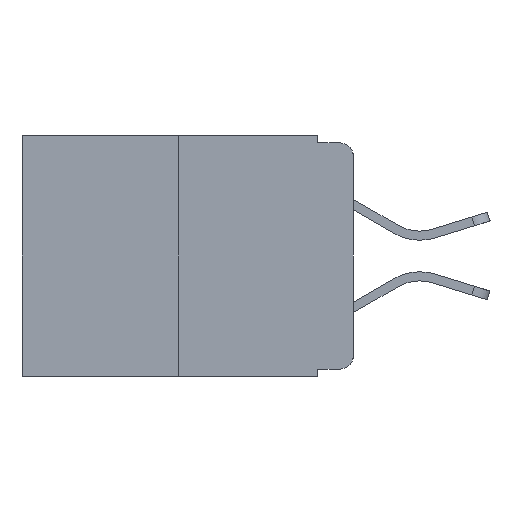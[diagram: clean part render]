
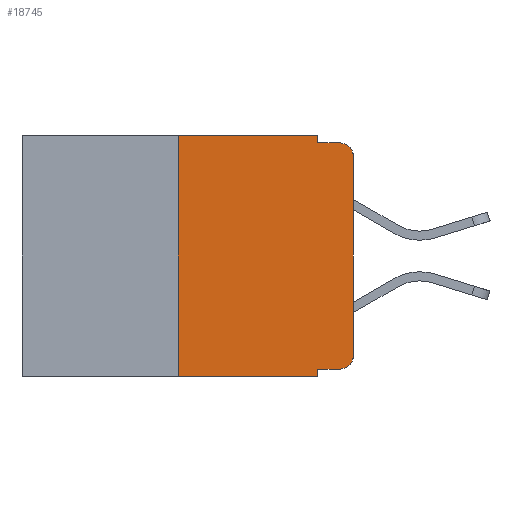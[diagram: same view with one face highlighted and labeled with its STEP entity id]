
A CAD part, left-side view. The second image highlights one B-rep face of the part: STEP entity #18745.
In plain terms, the highlighted planar face has unit normal (-1, 0, 0).
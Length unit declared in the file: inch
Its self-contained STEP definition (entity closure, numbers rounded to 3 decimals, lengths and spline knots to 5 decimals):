
#181 = EDGE_CURVE ( 'NONE', #6180, #10598, #3139, .T. ) ;
#533 = EDGE_CURVE ( 'NONE', #6180, #20550, #6608, .T. ) ;
#753 = LINE ( 'NONE', #8693, #20021 ) ;
#947 = DIRECTION ( 'NONE',  ( 0., 0., -1. ) ) ;
#1002 = ORIENTED_EDGE ( 'NONE', *, *, #10294, .T. ) ;
#1076 = VERTEX_POINT ( 'NONE', #17053 ) ;
#1227 = CARTESIAN_POINT ( 'NONE',  ( 0., 0.02, -0.313 ) ) ;
#2533 = CARTESIAN_POINT ( 'NONE',  ( 0., 0.051, 0. ) ) ;
#2749 = EDGE_CURVE ( 'NONE', #11808, #15245, #6987, .T. ) ;
#2962 = DIRECTION ( 'NONE',  ( 0., 0., 1. ) ) ;
#3079 = ORIENTED_EDGE ( 'NONE', *, *, #6478, .F. ) ;
#3130 = DIRECTION ( 'NONE',  ( 0., 0., -1. ) ) ;
#3139 = LINE ( 'NONE', #13725, #12553 ) ;
#3158 = AXIS2_PLACEMENT_3D ( 'NONE', #1227, #14376, #3130 ) ;
#3299 = LINE ( 'NONE', #3784, #22401 ) ;
#3784 = CARTESIAN_POINT ( 'NONE',  ( 0., 0.051, -0.01 ) ) ;
#4069 = LINE ( 'NONE', #22769, #8427 ) ;
#4880 = VECTOR ( 'NONE', #19027, 39.37008 ) ;
#5183 = DIRECTION ( 'NONE',  ( 0., 0., 1. ) ) ;
#6013 = ORIENTED_EDGE ( 'NONE', *, *, #20651, .T. ) ;
#6180 = VERTEX_POINT ( 'NONE', #21287 ) ;
#6381 = CARTESIAN_POINT ( 'NONE',  ( 0., 0.473, -0.343 ) ) ;
#6478 = EDGE_CURVE ( 'NONE', #15245, #23423, #3299, .T. ) ;
#6608 = LINE ( 'NONE', #6381, #4880 ) ;
#6987 = LINE ( 'NONE', #8072, #21183 ) ;
#7202 = ORIENTED_EDGE ( 'NONE', *, *, #23045, .F. ) ;
#8015 = DIRECTION ( 'NONE',  ( 0., 0., -1. ) ) ;
#8072 = CARTESIAN_POINT ( 'NONE',  ( 0., 0.051, 0. ) ) ;
#8427 = VECTOR ( 'NONE', #11898, 39.37008 ) ;
#8604 = CARTESIAN_POINT ( 'NONE',  ( 0., 0.051, -0.343 ) ) ;
#8693 = CARTESIAN_POINT ( 'NONE',  ( 0., 0.473, 0. ) ) ;
#8812 = AXIS2_PLACEMENT_3D ( 'NONE', #23156, #12225, #947 ) ;
#8959 = ORIENTED_EDGE ( 'NONE', *, *, #14393, .F. ) ;
#9006 = EDGE_CURVE ( 'NONE', #16203, #23423, #22796, .T. ) ;
#9014 = CIRCLE ( 'NONE', #3158, 0.02 ) ;
#9024 = CARTESIAN_POINT ( 'NONE',  ( 0., 0., -0.313 ) ) ;
#9317 = CARTESIAN_POINT ( 'NONE',  ( 0., 0.051, -0.01 ) ) ;
#9419 = FACE_OUTER_BOUND ( 'NONE', #19785, .T. ) ;
#9778 = VECTOR ( 'NONE', #2962, 39.37008 ) ;
#10030 = VERTEX_POINT ( 'NONE', #18888 ) ;
#10080 = PLANE ( 'NONE',  #20150 ) ;
#10155 = CARTESIAN_POINT ( 'NONE',  ( 0., 0.473, 0. ) ) ;
#10159 = ORIENTED_EDGE ( 'NONE', *, *, #2749, .F. ) ;
#10294 = EDGE_CURVE ( 'NONE', #16328, #16203, #20779, .T. ) ;
#10598 = VERTEX_POINT ( 'NONE', #23136 ) ;
#11808 = VERTEX_POINT ( 'NONE', #2533 ) ;
#11898 = DIRECTION ( 'NONE',  ( 0., -1., 0. ) ) ;
#12061 = DIRECTION ( 'NONE',  ( 0., 0., -1. ) ) ;
#12225 = DIRECTION ( 'NONE',  ( -1., 0., 0. ) ) ;
#12337 = CARTESIAN_POINT ( 'NONE',  ( 0., 0., 0. ) ) ;
#12519 = DIRECTION ( 'NONE',  ( 0., -1., 0. ) ) ;
#12553 = VECTOR ( 'NONE', #5183, 39.37008 ) ;
#12586 = CARTESIAN_POINT ( 'NONE',  ( 0., 0.02, -0.01 ) ) ;
#12827 = ORIENTED_EDGE ( 'NONE', *, *, #533, .T. ) ;
#13489 = DIRECTION ( 'NONE',  ( 0., 0., -1. ) ) ;
#13725 = CARTESIAN_POINT ( 'NONE',  ( 0., 0.25, 0. ) ) ;
#14376 = DIRECTION ( 'NONE',  ( -1., 0., 0. ) ) ;
#14393 = EDGE_CURVE ( 'NONE', #10598, #11808, #753, .T. ) ;
#15245 = VERTEX_POINT ( 'NONE', #9317 ) ;
#16203 = VERTEX_POINT ( 'NONE', #21548 ) ;
#16328 = VERTEX_POINT ( 'NONE', #9024 ) ;
#17053 = CARTESIAN_POINT ( 'NONE',  ( 0., 0.02, -0.333 ) ) ;
#17437 = VECTOR ( 'NONE', #13489, 39.37008 ) ;
#17756 = ORIENTED_EDGE ( 'NONE', *, *, #181, .F. ) ;
#18009 = LINE ( 'NONE', #20763, #17437 ) ;
#18250 = EDGE_CURVE ( 'NONE', #1076, #16328, #9014, .T. ) ;
#18745 = ADVANCED_FACE ( 'NONE', ( #9419 ), #10080, .F. ) ;
#18888 = CARTESIAN_POINT ( 'NONE',  ( 0., 0.051, -0.333 ) ) ;
#19027 = DIRECTION ( 'NONE',  ( 0., -1., 0. ) ) ;
#19785 = EDGE_LOOP ( 'NONE', ( #1002, #23882, #3079, #10159, #8959, #17756, #12827, #7202, #6013, #23344 ) ) ;
#20021 = VECTOR ( 'NONE', #12519, 39.37008 ) ;
#20150 = AXIS2_PLACEMENT_3D ( 'NONE', #10155, #23006, #12061 ) ;
#20504 = DIRECTION ( 'NONE',  ( 0., -1., 0. ) ) ;
#20550 = VERTEX_POINT ( 'NONE', #8604 ) ;
#20651 = EDGE_CURVE ( 'NONE', #10030, #1076, #4069, .T. ) ;
#20763 = CARTESIAN_POINT ( 'NONE',  ( 0., 0.051, 0. ) ) ;
#20779 = LINE ( 'NONE', #12337, #9778 ) ;
#21183 = VECTOR ( 'NONE', #8015, 39.37008 ) ;
#21287 = CARTESIAN_POINT ( 'NONE',  ( 0., 0.25, -0.343 ) ) ;
#21548 = CARTESIAN_POINT ( 'NONE',  ( 0., 0., -0.03 ) ) ;
#22401 = VECTOR ( 'NONE', #20504, 39.37008 ) ;
#22769 = CARTESIAN_POINT ( 'NONE',  ( 0., 0.051, -0.333 ) ) ;
#22796 = CIRCLE ( 'NONE', #8812, 0.02 ) ;
#23006 = DIRECTION ( 'NONE',  ( 1., 0., 0. ) ) ;
#23045 = EDGE_CURVE ( 'NONE', #10030, #20550, #18009, .T. ) ;
#23136 = CARTESIAN_POINT ( 'NONE',  ( 0., 0.25, 0. ) ) ;
#23156 = CARTESIAN_POINT ( 'NONE',  ( 0., 0.02, -0.03 ) ) ;
#23344 = ORIENTED_EDGE ( 'NONE', *, *, #18250, .T. ) ;
#23423 = VERTEX_POINT ( 'NONE', #12586 ) ;
#23882 = ORIENTED_EDGE ( 'NONE', *, *, #9006, .T. ) ;
